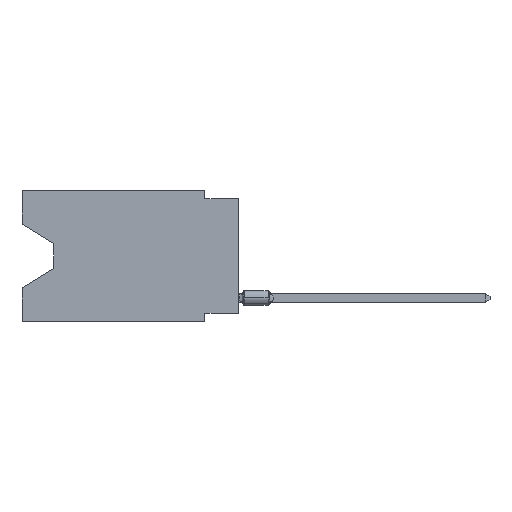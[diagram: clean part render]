
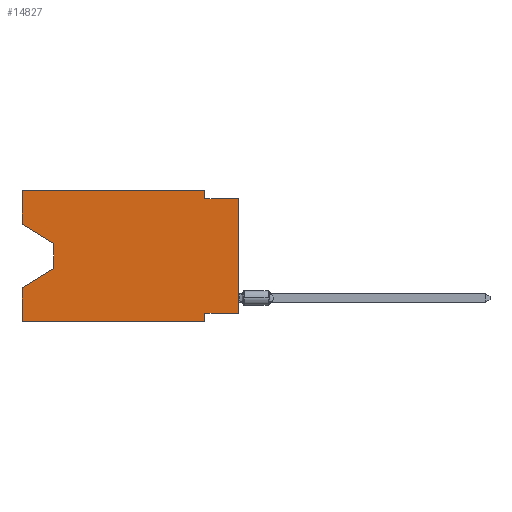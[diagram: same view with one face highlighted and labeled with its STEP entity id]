
A CAD part, left-side view. The second image highlights one B-rep face of the part: STEP entity #14827.
In plain terms, the highlighted planar face has unit normal (-1, 0, 0).
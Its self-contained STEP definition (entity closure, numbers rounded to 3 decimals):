
#34 = LINE ( 'NONE', #24317, #24671 ) ;
#235 = VECTOR ( 'NONE', #17558, 1000. ) ;
#535 = VECTOR ( 'NONE', #22741, 1000. ) ;
#1292 = CARTESIAN_POINT ( 'NONE',  ( 0., 2.54, -0.635 ) ) ;
#1575 = DIRECTION ( 'NONE',  ( 0., 1., 0. ) ) ;
#1579 = CARTESIAN_POINT ( 'NONE',  ( 0., 2.54, 0. ) ) ;
#1697 = VERTEX_POINT ( 'NONE', #27088 ) ;
#1941 = DIRECTION ( 'NONE',  ( 0., 0., 1. ) ) ;
#2099 = CARTESIAN_POINT ( 'NONE',  ( 0., 16.383, 0. ) ) ;
#2118 = VERTEX_POINT ( 'NONE', #1579 ) ;
#2432 = ORIENTED_EDGE ( 'NONE', *, *, #12217, .T. ) ;
#3052 = CARTESIAN_POINT ( 'NONE',  ( 0., 0., -9.271 ) ) ;
#3421 = VERTEX_POINT ( 'NONE', #11784 ) ;
#3526 = CARTESIAN_POINT ( 'NONE',  ( 0., 0., -9.271 ) ) ;
#3987 = CARTESIAN_POINT ( 'NONE',  ( 0., 16.383, 0. ) ) ;
#4115 = VECTOR ( 'NONE', #6467, 1000. ) ;
#4146 = ORIENTED_EDGE ( 'NONE', *, *, #15816, .F. ) ;
#4359 = CARTESIAN_POINT ( 'NONE',  ( 0., 0., 0. ) ) ;
#4543 = CARTESIAN_POINT ( 'NONE',  ( 0., 2.54, 0. ) ) ;
#4913 = LINE ( 'NONE', #29666, #25048 ) ;
#5033 = LINE ( 'NONE', #17347, #17435 ) ;
#5049 = VECTOR ( 'NONE', #1575, 1000. ) ;
#6364 = CARTESIAN_POINT ( 'NONE',  ( 0., 16.383, -9.906 ) ) ;
#6383 = DIRECTION ( 'NONE',  ( 0., 0., -1. ) ) ;
#6413 = VECTOR ( 'NONE', #22850, 1000. ) ;
#6467 = DIRECTION ( 'NONE',  ( 0., 0., 1. ) ) ;
#6728 = FACE_OUTER_BOUND ( 'NONE', #28661, .T. ) ;
#6847 = ORIENTED_EDGE ( 'NONE', *, *, #27483, .T. ) ;
#7052 = DIRECTION ( 'NONE',  ( 1., 0., 0. ) ) ;
#7064 = ORIENTED_EDGE ( 'NONE', *, *, #16661, .T. ) ;
#7666 = CARTESIAN_POINT ( 'NONE',  ( 0., 13.97, -5.893 ) ) ;
#9415 = CARTESIAN_POINT ( 'NONE',  ( 0., 13.97, -4.013 ) ) ;
#9768 = ORIENTED_EDGE ( 'NONE', *, *, #20289, .F. ) ;
#9855 = EDGE_CURVE ( 'NONE', #20098, #18701, #16502, .T. ) ;
#10854 = VERTEX_POINT ( 'NONE', #6364 ) ;
#11784 = CARTESIAN_POINT ( 'NONE',  ( 0., 13.97, -5.893 ) ) ;
#12190 = EDGE_CURVE ( 'NONE', #15740, #2118, #4913, .T. ) ;
#12217 = EDGE_CURVE ( 'NONE', #3421, #19474, #22109, .T. ) ;
#12305 = ORIENTED_EDGE ( 'NONE', *, *, #9855, .T. ) ;
#12549 = CARTESIAN_POINT ( 'NONE',  ( 0., 16.383, -7.36 ) ) ;
#13191 = VERTEX_POINT ( 'NONE', #1292 ) ;
#13684 = ORIENTED_EDGE ( 'NONE', *, *, #12190, .F. ) ;
#14004 = ORIENTED_EDGE ( 'NONE', *, *, #23477, .F. ) ;
#14590 = LINE ( 'NONE', #4543, #31182 ) ;
#14715 = VECTOR ( 'NONE', #28618, 1000. ) ;
#14805 = DIRECTION ( 'NONE',  ( 0., -1., 0. ) ) ;
#14827 = ADVANCED_FACE ( 'NONE', ( #6728 ), #17105, .F. ) ;
#15740 = VERTEX_POINT ( 'NONE', #22356 ) ;
#15816 = EDGE_CURVE ( 'NONE', #2118, #13191, #14590, .T. ) ;
#16111 = ORIENTED_EDGE ( 'NONE', *, *, #26790, .F. ) ;
#16502 = LINE ( 'NONE', #31044, #14715 ) ;
#16661 = EDGE_CURVE ( 'NONE', #18701, #3421, #23336, .T. ) ;
#16944 = DIRECTION ( 'NONE',  ( 0., 0., -1. ) ) ;
#17105 = PLANE ( 'NONE',  #20027 ) ;
#17347 = CARTESIAN_POINT ( 'NONE',  ( 0., 0., -0.635 ) ) ;
#17435 = VECTOR ( 'NONE', #31900, 1000. ) ;
#17558 = DIRECTION ( 'NONE',  ( 0., 0.855, -0.519 ) ) ;
#17668 = DIRECTION ( 'NONE',  ( 0., -1., 0. ) ) ;
#17861 = CARTESIAN_POINT ( 'NONE',  ( 0., 2.54, -9.906 ) ) ;
#18581 = LINE ( 'NONE', #21166, #29255 ) ;
#18701 = VERTEX_POINT ( 'NONE', #9415 ) ;
#18796 = LINE ( 'NONE', #4359, #4115 ) ;
#19077 = CARTESIAN_POINT ( 'NONE',  ( 0., 2.54, -9.271 ) ) ;
#19123 = LINE ( 'NONE', #2099, #29640 ) ;
#19474 = VERTEX_POINT ( 'NONE', #12549 ) ;
#20027 = AXIS2_PLACEMENT_3D ( 'NONE', #3987, #7052, #16944 ) ;
#20098 = VERTEX_POINT ( 'NONE', #25755 ) ;
#20289 = EDGE_CURVE ( 'NONE', #28907, #24154, #18581, .T. ) ;
#20907 = CARTESIAN_POINT ( 'NONE',  ( 0., 13.97, -4.013 ) ) ;
#21166 = CARTESIAN_POINT ( 'NONE',  ( 0., 2.54, -9.906 ) ) ;
#22044 = DIRECTION ( 'NONE',  ( 0., 0., -1. ) ) ;
#22109 = LINE ( 'NONE', #7666, #235 ) ;
#22356 = CARTESIAN_POINT ( 'NONE',  ( 0., 16.383, 0. ) ) ;
#22741 = DIRECTION ( 'NONE',  ( 0., 0., 1. ) ) ;
#22850 = DIRECTION ( 'NONE',  ( 0., 0., -1. ) ) ;
#23115 = EDGE_CURVE ( 'NONE', #10854, #24154, #34, .T. ) ;
#23336 = LINE ( 'NONE', #20907, #6413 ) ;
#23477 = EDGE_CURVE ( 'NONE', #10854, #19474, #19123, .T. ) ;
#23766 = LINE ( 'NONE', #3526, #5049 ) ;
#24154 = VERTEX_POINT ( 'NONE', #17861 ) ;
#24317 = CARTESIAN_POINT ( 'NONE',  ( 0., 16.383, -9.906 ) ) ;
#24671 = VECTOR ( 'NONE', #17668, 1000. ) ;
#24974 = ORIENTED_EDGE ( 'NONE', *, *, #30042, .F. ) ;
#25048 = VECTOR ( 'NONE', #14805, 1000. ) ;
#25556 = ORIENTED_EDGE ( 'NONE', *, *, #29395, .F. ) ;
#25755 = CARTESIAN_POINT ( 'NONE',  ( 0., 16.383, -2.546 ) ) ;
#26790 = EDGE_CURVE ( 'NONE', #20098, #15740, #27739, .T. ) ;
#26830 = CARTESIAN_POINT ( 'NONE',  ( 0., 16.383, 0. ) ) ;
#27088 = CARTESIAN_POINT ( 'NONE',  ( 0., 0., -0.635 ) ) ;
#27483 = EDGE_CURVE ( 'NONE', #31850, #1697, #18796, .T. ) ;
#27739 = LINE ( 'NONE', #26830, #535 ) ;
#28618 = DIRECTION ( 'NONE',  ( 0., -0.855, -0.519 ) ) ;
#28661 = EDGE_LOOP ( 'NONE', ( #12305, #7064, #2432, #14004, #28849, #9768, #24974, #6847, #25556, #4146, #13684, #16111 ) ) ;
#28849 = ORIENTED_EDGE ( 'NONE', *, *, #23115, .T. ) ;
#28907 = VERTEX_POINT ( 'NONE', #19077 ) ;
#29255 = VECTOR ( 'NONE', #6383, 1000. ) ;
#29395 = EDGE_CURVE ( 'NONE', #13191, #1697, #5033, .T. ) ;
#29640 = VECTOR ( 'NONE', #1941, 1000. ) ;
#29666 = CARTESIAN_POINT ( 'NONE',  ( 0., 16.383, 0. ) ) ;
#30042 = EDGE_CURVE ( 'NONE', #31850, #28907, #23766, .T. ) ;
#31044 = CARTESIAN_POINT ( 'NONE',  ( 0., 16.383, -2.546 ) ) ;
#31182 = VECTOR ( 'NONE', #22044, 1000. ) ;
#31850 = VERTEX_POINT ( 'NONE', #3052 ) ;
#31900 = DIRECTION ( 'NONE',  ( 0., -1., 0. ) ) ;
